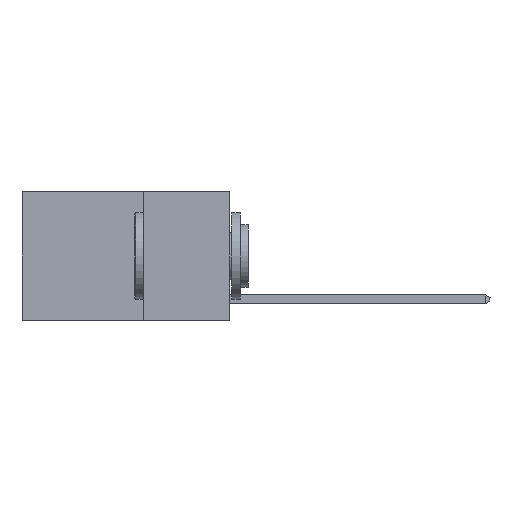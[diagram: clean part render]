
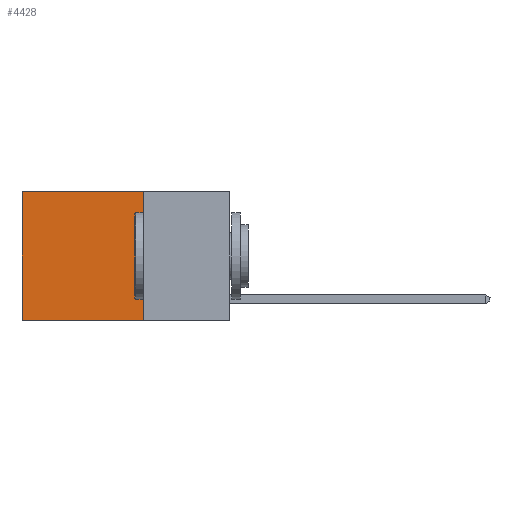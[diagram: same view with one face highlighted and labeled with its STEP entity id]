
A CAD part, left-side view. The second image highlights one B-rep face of the part: STEP entity #4428.
In plain terms, the highlighted planar face has unit normal (-1, 0, 0).
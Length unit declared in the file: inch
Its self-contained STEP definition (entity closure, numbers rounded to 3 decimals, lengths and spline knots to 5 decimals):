
#353 = EDGE_CURVE ( 'NONE', #7818, #3652, #7966, .T. ) ;
#1266 = EDGE_LOOP ( 'NONE', ( #4660, #22391, #24048, #6254 ) ) ;
#2133 = CARTESIAN_POINT ( 'NONE',  ( 0.2625, 0.25, 0. ) ) ;
#2758 = VECTOR ( 'NONE', #9745, 39.37008 ) ;
#3279 = CARTESIAN_POINT ( 'NONE',  ( 0.2625, 0.25, 0. ) ) ;
#3643 = DIRECTION ( 'NONE',  ( 1., 0., 0. ) ) ;
#3652 = VERTEX_POINT ( 'NONE', #15746 ) ;
#3957 = VECTOR ( 'NONE', #17889, 39.37008 ) ;
#4428 = ADVANCED_FACE ( 'NONE', ( #20437 ), #23896, .F. ) ;
#4660 = ORIENTED_EDGE ( 'NONE', *, *, #21487, .T. ) ;
#6254 = ORIENTED_EDGE ( 'NONE', *, *, #21848, .T. ) ;
#7313 = CARTESIAN_POINT ( 'NONE',  ( 0.2625, 0.6, -0.37 ) ) ;
#7818 = VERTEX_POINT ( 'NONE', #16374 ) ;
#7966 = LINE ( 'NONE', #8088, #12831 ) ;
#8088 = CARTESIAN_POINT ( 'NONE',  ( 0.2625, 0.25, 0. ) ) ;
#9745 = DIRECTION ( 'NONE',  ( 0., 0., -1. ) ) ;
#11731 = VECTOR ( 'NONE', #20779, 39.37008 ) ;
#12365 = AXIS2_PLACEMENT_3D ( 'NONE', #3279, #3643, #18588 ) ;
#12831 = VECTOR ( 'NONE', #15474, 39.37008 ) ;
#13270 = LINE ( 'NONE', #2133, #11731 ) ;
#13480 = CARTESIAN_POINT ( 'NONE',  ( 0.2625, 0.6, 0. ) ) ;
#14325 = VERTEX_POINT ( 'NONE', #17774 ) ;
#15474 = DIRECTION ( 'NONE',  ( 0., 0., -1. ) ) ;
#15746 = CARTESIAN_POINT ( 'NONE',  ( 0.2625, 0.25, -0.37 ) ) ;
#16374 = CARTESIAN_POINT ( 'NONE',  ( 0.2625, 0.25, 0. ) ) ;
#16609 = VERTEX_POINT ( 'NONE', #7313 ) ;
#17138 = LINE ( 'NONE', #13480, #2758 ) ;
#17774 = CARTESIAN_POINT ( 'NONE',  ( 0.2625, 0.6, 0. ) ) ;
#17889 = DIRECTION ( 'NONE',  ( 0., 1., 0. ) ) ;
#18588 = DIRECTION ( 'NONE',  ( 0., 0., -1. ) ) ;
#20008 = CARTESIAN_POINT ( 'NONE',  ( 0.2625, 0.25, -0.37 ) ) ;
#20437 = FACE_OUTER_BOUND ( 'NONE', #1266, .T. ) ;
#20779 = DIRECTION ( 'NONE',  ( 0., 1., 0. ) ) ;
#21337 = EDGE_CURVE ( 'NONE', #3652, #16609, #21743, .T. ) ;
#21487 = EDGE_CURVE ( 'NONE', #14325, #16609, #17138, .T. ) ;
#21743 = LINE ( 'NONE', #20008, #3957 ) ;
#21848 = EDGE_CURVE ( 'NONE', #7818, #14325, #13270, .T. ) ;
#22391 = ORIENTED_EDGE ( 'NONE', *, *, #21337, .F. ) ;
#23896 = PLANE ( 'NONE',  #12365 ) ;
#24048 = ORIENTED_EDGE ( 'NONE', *, *, #353, .F. ) ;
